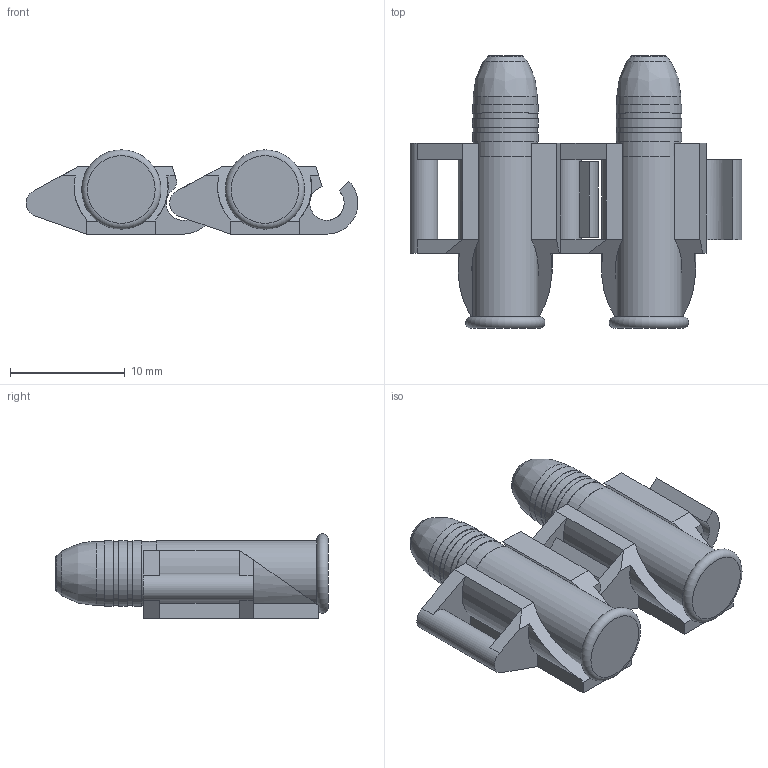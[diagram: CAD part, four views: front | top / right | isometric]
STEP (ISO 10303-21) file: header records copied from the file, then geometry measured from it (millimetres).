
FILE_DESCRIPTION(/* description */ (''),/* implementation_level */ '2;1');
FILE_NAME(/* name */ 'links.stp',/* time_stamp */ '2021-07-16T21:38:59+02:00',/* author */ (''),/* organization */ (''),/* preprocessor_version */ 'ST-DEVELOPER v15.2',/* originating_system */ 'Autodesk Translator Framework v2.0.0.5431',/* authorisation */ '');
FILE_SCHEMA (('AUTOMOTIVE_DESIGN { 1 0 10303 214 3 1 1 }'));
Length unit declared in the file: centimetre
Products named in the file (1): (Unsaved)
Bounding box: 28.89 x 23.75 x 7.34 mm (x, y, z)
Volume: 2007.5 mm3; surface area: 2412.4 mm2
Topology: 4 solids, 4 shells, 115 faces, 258 edges, 165 vertices
Faces by surface type: plane 70, cylinder 33, torus 6, bspline 2, sphere 2, cone 2
Full cylindrical faces by diameter (mm): 0.793 x2, 2.4 x2, 5.588 x8, 5.69 x2, 5.715 x6
Entity records: 3139 total; most frequent: CARTESIAN_POINT 577, DIRECTION 550, ORIENTED_EDGE 464, EDGE_CURVE 232, AXIS2_PLACEMENT_3D 210, VERTEX_POINT 165, EDGE_LOOP 159, LINE 130
